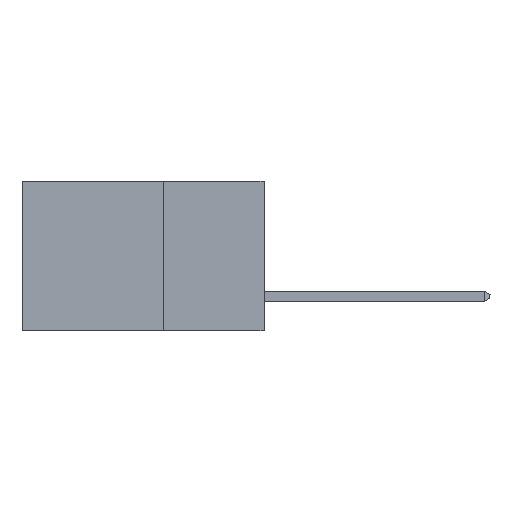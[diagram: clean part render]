
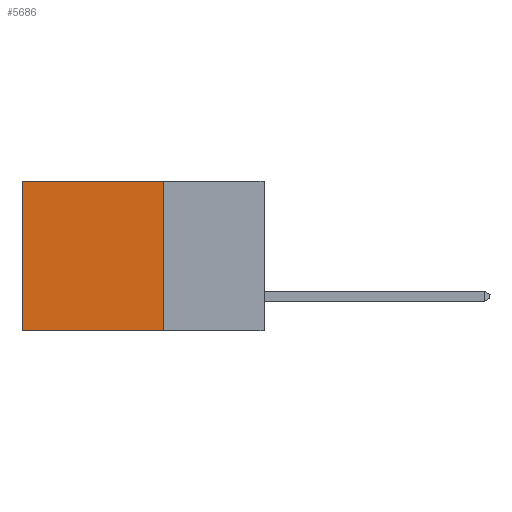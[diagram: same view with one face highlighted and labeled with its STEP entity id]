
A CAD part, left-side view. The second image highlights one B-rep face of the part: STEP entity #5686.
In plain terms, the highlighted planar face has unit normal (-1, 0, 0).
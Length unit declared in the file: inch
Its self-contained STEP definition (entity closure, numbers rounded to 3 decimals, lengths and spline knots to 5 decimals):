
#84 = CARTESIAN_POINT ( 'NONE',  ( 0.298, 0.25, -0.37 ) ) ;
#311 = DIRECTION ( 'NONE',  ( 0., 0., -1. ) ) ;
#488 = EDGE_CURVE ( 'NONE', #8701, #4116, #813, .T. ) ;
#813 = LINE ( 'NONE', #3204, #7987 ) ;
#959 = EDGE_CURVE ( 'NONE', #9021, #4116, #3450, .T. ) ;
#1027 = CARTESIAN_POINT ( 'NONE',  ( 0.298, 0.25, 0. ) ) ;
#1071 = EDGE_CURVE ( 'NONE', #4289, #8701, #4596, .T. ) ;
#1335 = DIRECTION ( 'NONE',  ( 0., 0., -1. ) ) ;
#1362 = EDGE_CURVE ( 'NONE', #4289, #9021, #4900, .T. ) ;
#1781 = CARTESIAN_POINT ( 'NONE',  ( 0.298, 0.6, -0.37 ) ) ;
#2197 = AXIS2_PLACEMENT_3D ( 'NONE', #7713, #8494, #2956 ) ;
#2260 = VECTOR ( 'NONE', #2656, 39.37008 ) ;
#2262 = ORIENTED_EDGE ( 'NONE', *, *, #1362, .F. ) ;
#2656 = DIRECTION ( 'NONE',  ( 0., 1., 0. ) ) ;
#2927 = DIRECTION ( 'NONE',  ( 0., 1., 0. ) ) ;
#2956 = DIRECTION ( 'NONE',  ( 0., 0., -1. ) ) ;
#3204 = CARTESIAN_POINT ( 'NONE',  ( 0.298, 0.6, 0. ) ) ;
#3450 = LINE ( 'NONE', #84, #2260 ) ;
#4116 = VERTEX_POINT ( 'NONE', #1781 ) ;
#4289 = VERTEX_POINT ( 'NONE', #10623 ) ;
#4483 = ORIENTED_EDGE ( 'NONE', *, *, #488, .T. ) ;
#4596 = LINE ( 'NONE', #1027, #5791 ) ;
#4900 = LINE ( 'NONE', #7873, #9613 ) ;
#5686 = ADVANCED_FACE ( 'NONE', ( #11334 ), #8538, .F. ) ;
#5791 = VECTOR ( 'NONE', #2927, 39.37008 ) ;
#5855 = ORIENTED_EDGE ( 'NONE', *, *, #959, .F. ) ;
#6587 = CARTESIAN_POINT ( 'NONE',  ( 0.298, 0.6, 0. ) ) ;
#7713 = CARTESIAN_POINT ( 'NONE',  ( 0.298, 0.25, 0. ) ) ;
#7873 = CARTESIAN_POINT ( 'NONE',  ( 0.298, 0.25, 0. ) ) ;
#7987 = VECTOR ( 'NONE', #1335, 39.37008 ) ;
#8273 = CARTESIAN_POINT ( 'NONE',  ( 0.298, 0.25, -0.37 ) ) ;
#8494 = DIRECTION ( 'NONE',  ( 1., 0., 0. ) ) ;
#8538 = PLANE ( 'NONE',  #2197 ) ;
#8701 = VERTEX_POINT ( 'NONE', #6587 ) ;
#9021 = VERTEX_POINT ( 'NONE', #8273 ) ;
#9613 = VECTOR ( 'NONE', #311, 39.37008 ) ;
#10623 = CARTESIAN_POINT ( 'NONE',  ( 0.298, 0.25, 0. ) ) ;
#11091 = ORIENTED_EDGE ( 'NONE', *, *, #1071, .T. ) ;
#11334 = FACE_OUTER_BOUND ( 'NONE', #12078, .T. ) ;
#12078 = EDGE_LOOP ( 'NONE', ( #4483, #5855, #2262, #11091 ) ) ;
